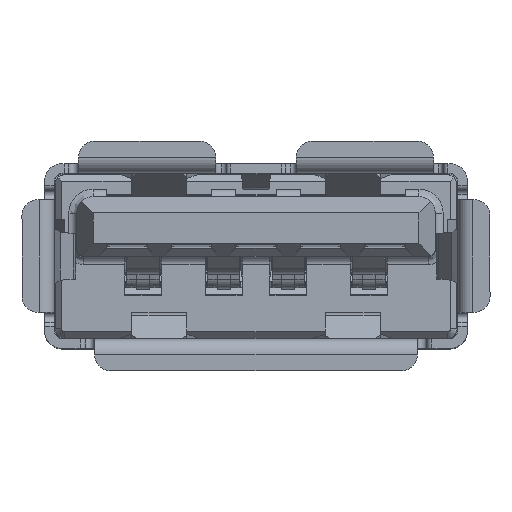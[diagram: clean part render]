
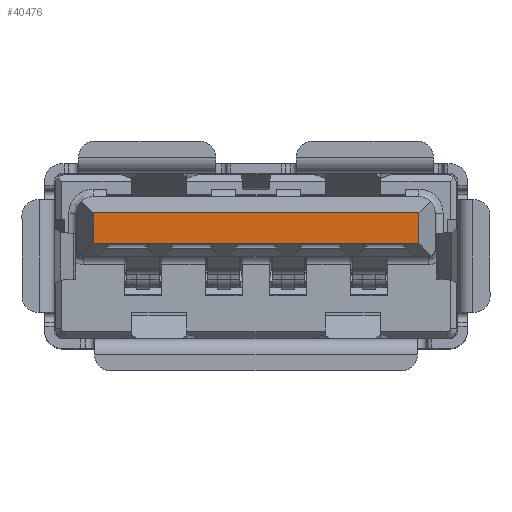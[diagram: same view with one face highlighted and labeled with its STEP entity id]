
A CAD part, top view. The second image highlights one B-rep face of the part: STEP entity #40476.
In plain terms, the highlighted face is planar.
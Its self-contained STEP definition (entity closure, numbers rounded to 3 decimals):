
#1135 = DIRECTION ( 'NONE',  ( -1., 0., 0. ) ) ;
#2142 = CARTESIAN_POINT ( 'NONE',  ( 0., -10.25, -0.38 ) ) ;
#3485 = EDGE_CURVE ( 'NONE', #25927, #46388, #34218, .T. ) ;
#4915 = LINE ( 'NONE', #40269, #35189 ) ;
#5192 = PLANE ( 'NONE',  #35195 ) ;
#8105 = CARTESIAN_POINT ( 'NONE',  ( 0., -10.25, -1.34 ) ) ;
#11348 = VECTOR ( 'NONE', #19831, 1000. ) ;
#13772 = VERTEX_POINT ( 'NONE', #41443 ) ;
#14314 = ORIENTED_EDGE ( 'NONE', *, *, #3485, .T. ) ;
#17585 = EDGE_CURVE ( 'NONE', #13772, #25927, #50354, .T. ) ;
#18260 = VECTOR ( 'NONE', #54975, 1000. ) ;
#18837 = DIRECTION ( 'NONE',  ( 0., 0., 1. ) ) ;
#19087 = CARTESIAN_POINT ( 'NONE',  ( -5.05, -10.25, -0.86 ) ) ;
#19831 = DIRECTION ( 'NONE',  ( -1., 0., 0. ) ) ;
#24834 = EDGE_CURVE ( 'NONE', #46388, #32877, #4915, .T. ) ;
#25380 = CARTESIAN_POINT ( 'NONE',  ( 5.05, -10.25, -1.34 ) ) ;
#25927 = VERTEX_POINT ( 'NONE', #35365 ) ;
#31851 = ORIENTED_EDGE ( 'NONE', *, *, #24834, .T. ) ;
#31878 = DIRECTION ( 'NONE',  ( 0., -1., 0. ) ) ;
#32877 = VERTEX_POINT ( 'NONE', #45268 ) ;
#34218 = LINE ( 'NONE', #8105, #48571 ) ;
#35189 = VECTOR ( 'NONE', #18837, 1000. ) ;
#35195 = AXIS2_PLACEMENT_3D ( 'NONE', #45482, #31878, #1135 ) ;
#35365 = CARTESIAN_POINT ( 'NONE',  ( -5.05, -10.25, -1.34 ) ) ;
#37790 = LINE ( 'NONE', #2142, #11348 ) ;
#37822 = EDGE_CURVE ( 'NONE', #32877, #13772, #37790, .T. ) ;
#39934 = ORIENTED_EDGE ( 'NONE', *, *, #37822, .T. ) ;
#40269 = CARTESIAN_POINT ( 'NONE',  ( 5.05, -10.25, -0.86 ) ) ;
#40476 = ADVANCED_FACE ( 'NONE', ( #54151 ), #5192, .T. ) ;
#41443 = CARTESIAN_POINT ( 'NONE',  ( -5.05, -10.25, -0.38 ) ) ;
#44832 = ORIENTED_EDGE ( 'NONE', *, *, #17585, .T. ) ;
#45268 = CARTESIAN_POINT ( 'NONE',  ( 5.05, -10.25, -0.38 ) ) ;
#45482 = CARTESIAN_POINT ( 'NONE',  ( 5.252, -10.25, -0.355 ) ) ;
#46388 = VERTEX_POINT ( 'NONE', #25380 ) ;
#48296 = EDGE_LOOP ( 'NONE', ( #39934, #44832, #14314, #31851 ) ) ;
#48571 = VECTOR ( 'NONE', #51878, 1000. ) ;
#50354 = LINE ( 'NONE', #19087, #18260 ) ;
#51878 = DIRECTION ( 'NONE',  ( 1., 0., 0. ) ) ;
#54151 = FACE_OUTER_BOUND ( 'NONE', #48296, .T. ) ;
#54975 = DIRECTION ( 'NONE',  ( 0., 0., -1. ) ) ;
